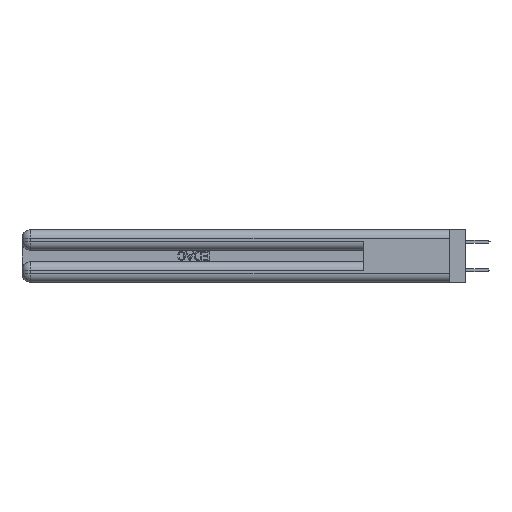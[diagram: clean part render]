
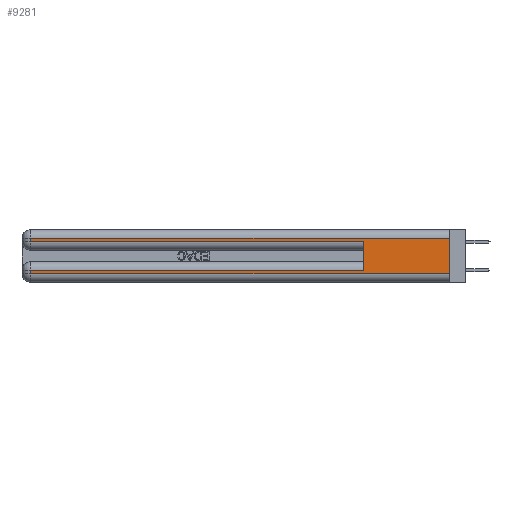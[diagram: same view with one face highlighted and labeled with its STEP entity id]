
A CAD part, left-side view. The second image highlights one B-rep face of the part: STEP entity #9281.
In plain terms, the highlighted planar face has unit normal (-1, 0, 0).
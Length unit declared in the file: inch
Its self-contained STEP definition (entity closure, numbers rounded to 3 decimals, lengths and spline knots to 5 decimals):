
#179 = EDGE_CURVE ( 'NONE', #20829, #34013, #36000, .T. ) ;
#285 = LINE ( 'NONE', #4840, #15823 ) ;
#495 = CARTESIAN_POINT ( 'NONE',  ( 0., 0., 0.37 ) ) ;
#540 = ORIENTED_EDGE ( 'NONE', *, *, #4765, .T. ) ;
#1086 = CARTESIAN_POINT ( 'NONE',  ( 0., 0., 0.31 ) ) ;
#1691 = LINE ( 'NONE', #30322, #4090 ) ;
#1753 = VERTEX_POINT ( 'NONE', #38419 ) ;
#2222 = EDGE_CURVE ( 'NONE', #20829, #19554, #2955, .T. ) ;
#2391 = DIRECTION ( 'NONE',  ( 0., 1., 0. ) ) ;
#2955 = LINE ( 'NONE', #11579, #5291 ) ;
#3480 = AXIS2_PLACEMENT_3D ( 'NONE', #495, #6000, #36857 ) ;
#4090 = VECTOR ( 'NONE', #9470, 39.37008 ) ;
#4199 = EDGE_CURVE ( 'NONE', #11510, #9206, #24877, .T. ) ;
#4765 = EDGE_CURVE ( 'NONE', #19554, #28548, #31841, .T. ) ;
#4840 = CARTESIAN_POINT ( 'NONE',  ( 0., 0., 0.085 ) ) ;
#5291 = VECTOR ( 'NONE', #34697, 39.37008 ) ;
#5443 = EDGE_CURVE ( 'NONE', #20254, #11510, #285, .T. ) ;
#6000 = DIRECTION ( 'NONE',  ( 1., 0., 0. ) ) ;
#7220 = ORIENTED_EDGE ( 'NONE', *, *, #21350, .F. ) ;
#8472 = ORIENTED_EDGE ( 'NONE', *, *, #5443, .T. ) ;
#9206 = VERTEX_POINT ( 'NONE', #37905 ) ;
#9281 = ADVANCED_FACE ( 'NONE', ( #32134 ), #14508, .F. ) ;
#9325 = VECTOR ( 'NONE', #19103, 39.37008 ) ;
#9397 = VECTOR ( 'NONE', #13637, 39.37008 ) ;
#9470 = DIRECTION ( 'NONE',  ( 0., -1., 0. ) ) ;
#10451 = DIRECTION ( 'NONE',  ( 0., -1., 0. ) ) ;
#11510 = VERTEX_POINT ( 'NONE', #31374 ) ;
#11579 = CARTESIAN_POINT ( 'NONE',  ( 0., 0., 0.31 ) ) ;
#13637 = DIRECTION ( 'NONE',  ( 0., 0., -1. ) ) ;
#14249 = CARTESIAN_POINT ( 'NONE',  ( 0., 0., 0.37 ) ) ;
#14508 = PLANE ( 'NONE',  #3480 ) ;
#15823 = VECTOR ( 'NONE', #2391, 39.37008 ) ;
#15839 = CARTESIAN_POINT ( 'NONE',  ( 0., 2.94, 0.31 ) ) ;
#19103 = DIRECTION ( 'NONE',  ( 0., 0., -1. ) ) ;
#19554 = VERTEX_POINT ( 'NONE', #15839 ) ;
#20254 = VERTEX_POINT ( 'NONE', #25619 ) ;
#20829 = VERTEX_POINT ( 'NONE', #1086 ) ;
#21350 = EDGE_CURVE ( 'NONE', #20254, #1753, #27938, .T. ) ;
#23537 = LINE ( 'NONE', #31572, #30091 ) ;
#23896 = ORIENTED_EDGE ( 'NONE', *, *, #34882, .T. ) ;
#24877 = LINE ( 'NONE', #31750, #9397 ) ;
#25255 = ORIENTED_EDGE ( 'NONE', *, *, #4199, .T. ) ;
#25619 = CARTESIAN_POINT ( 'NONE',  ( 0., 0.6, 0.085 ) ) ;
#27163 = DIRECTION ( 'NONE',  ( 0., 0., 1. ) ) ;
#27332 = EDGE_LOOP ( 'NONE', ( #29194, #32789, #540, #23896, #7220, #8472, #25255, #31689 ) ) ;
#27456 = VECTOR ( 'NONE', #27163, 39.37008 ) ;
#27485 = CARTESIAN_POINT ( 'NONE',  ( 0., 0., 0.06 ) ) ;
#27938 = LINE ( 'NONE', #33341, #27456 ) ;
#28548 = VERTEX_POINT ( 'NONE', #38004 ) ;
#29194 = ORIENTED_EDGE ( 'NONE', *, *, #179, .F. ) ;
#29814 = VECTOR ( 'NONE', #31962, 39.37008 ) ;
#30091 = VECTOR ( 'NONE', #10451, 39.37008 ) ;
#30322 = CARTESIAN_POINT ( 'NONE',  ( 0., 0., 0.06 ) ) ;
#31374 = CARTESIAN_POINT ( 'NONE',  ( 0., 2.94, 0.085 ) ) ;
#31572 = CARTESIAN_POINT ( 'NONE',  ( 0., 0., 0.285 ) ) ;
#31689 = ORIENTED_EDGE ( 'NONE', *, *, #36702, .T. ) ;
#31750 = CARTESIAN_POINT ( 'NONE',  ( 0., 2.94, 0.37 ) ) ;
#31841 = LINE ( 'NONE', #37021, #9325 ) ;
#31962 = DIRECTION ( 'NONE',  ( 0., 0., -1. ) ) ;
#32134 = FACE_OUTER_BOUND ( 'NONE', #27332, .T. ) ;
#32789 = ORIENTED_EDGE ( 'NONE', *, *, #2222, .T. ) ;
#33341 = CARTESIAN_POINT ( 'NONE',  ( 0., 0.6, 0.145 ) ) ;
#34013 = VERTEX_POINT ( 'NONE', #27485 ) ;
#34697 = DIRECTION ( 'NONE',  ( 0., 1., 0. ) ) ;
#34882 = EDGE_CURVE ( 'NONE', #28548, #1753, #23537, .T. ) ;
#36000 = LINE ( 'NONE', #14249, #29814 ) ;
#36702 = EDGE_CURVE ( 'NONE', #9206, #34013, #1691, .T. ) ;
#36857 = DIRECTION ( 'NONE',  ( 0., 0., -1. ) ) ;
#37021 = CARTESIAN_POINT ( 'NONE',  ( 0., 2.94, 0.37 ) ) ;
#37905 = CARTESIAN_POINT ( 'NONE',  ( 0., 2.94, 0.06 ) ) ;
#38004 = CARTESIAN_POINT ( 'NONE',  ( 0., 2.94, 0.285 ) ) ;
#38419 = CARTESIAN_POINT ( 'NONE',  ( 0., 0.6, 0.285 ) ) ;
